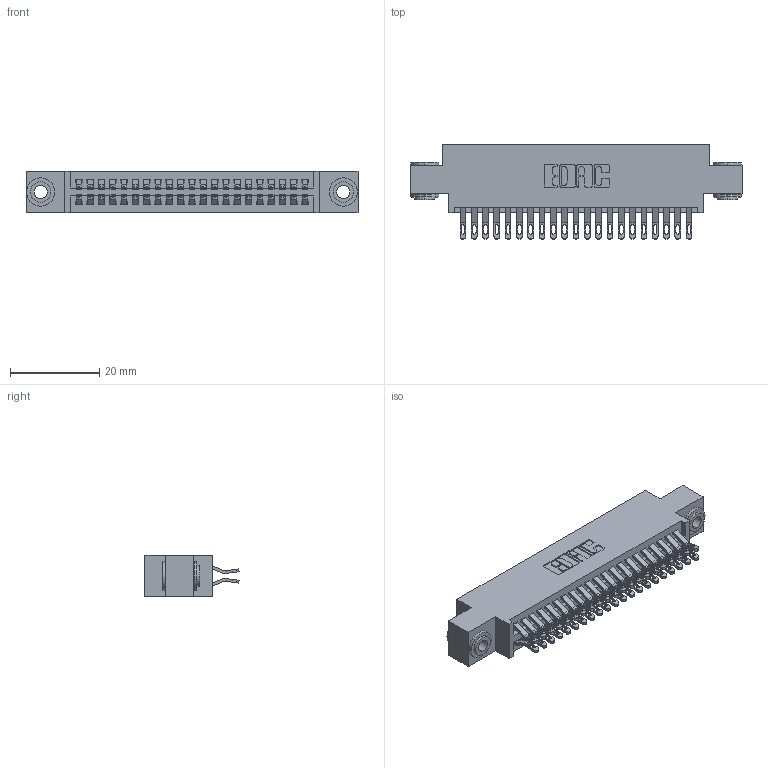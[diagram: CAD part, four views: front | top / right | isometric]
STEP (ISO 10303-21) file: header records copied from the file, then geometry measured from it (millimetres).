
FILE_DESCRIPTION (( 'STEP AP203' ), '1' );
FILE_NAME ('345-042-555-803.STEP', '2019-10-28T20:54:23', ( '' ), ( '' ), 'SwSTEP 2.0', 'SolidWorks 2016', '' );
FILE_SCHEMA (( 'CONFIG_CONTROL_DESIGN' ));
Length unit declared in the file: inch
Products named in the file (4): 345-042-555-803; 345-250-002_345-250-002-102; 345-292-001_555 Tail; 345 Part_0.170 Offset - 0.156 Dia-TH
Assembly tree (45 placements, depth 2):
  345-042-555-803
    345 Part_0.170 Offset - 0.156 Dia-TH
    345-292-001_555 Tail  x42
    345-250-002_345-250-002-102  x2
Bounding box: 74.55 x 21.13 x 9.4 mm (x, y, z)
Volume: 7074.7 mm3; surface area: 10822.9 mm2
Topology: 45 solids, 45 shells, 2520 faces, 7863 edges, 5238 vertices
Faces by surface type: plane 1396, cylinder 1116, cone 8
Entity records: 20412 total; most frequent: CARTESIAN_POINT 3453, ORIENTED_EDGE 3350, DIRECTION 3069, EDGE_CURVE 1675, VECTOR 1415, LINE 1415, VERTEX_POINT 1114, AXIS2_PLACEMENT_3D 827
